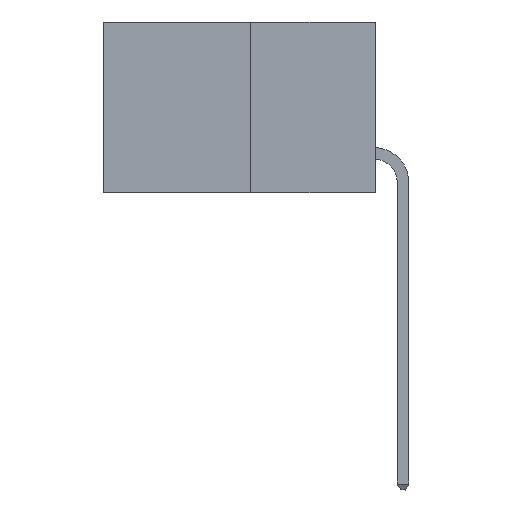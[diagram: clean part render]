
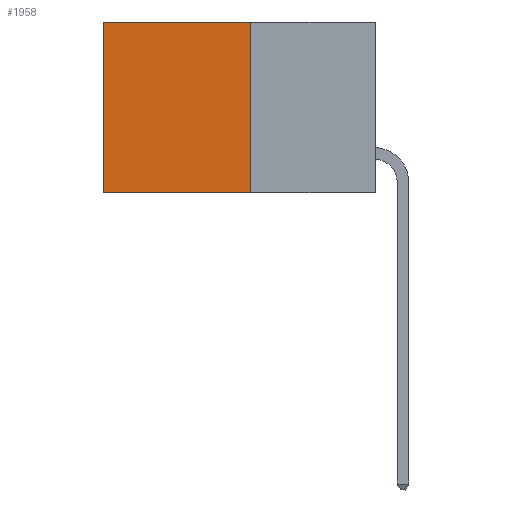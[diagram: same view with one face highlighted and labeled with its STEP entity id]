
A CAD part, left-side view. The second image highlights one B-rep face of the part: STEP entity #1958.
In plain terms, the highlighted planar face has unit normal (-1, 0, 0).
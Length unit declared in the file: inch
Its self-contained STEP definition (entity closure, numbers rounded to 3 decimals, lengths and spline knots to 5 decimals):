
#136 = EDGE_CURVE ( 'NONE', #5969, #7157, #6439, .T. ) ;
#255 = DIRECTION ( 'NONE',  ( 0., 0., -1. ) ) ;
#312 = VECTOR ( 'NONE', #472, 39.37008 ) ;
#472 = DIRECTION ( 'NONE',  ( 0., 0., -1. ) ) ;
#627 = VECTOR ( 'NONE', #8497, 39.37008 ) ;
#854 = VECTOR ( 'NONE', #8159, 39.37008 ) ;
#1305 = LINE ( 'NONE', #4364, #5028 ) ;
#1494 = EDGE_LOOP ( 'NONE', ( #1782, #3955, #5786, #7484 ) ) ;
#1782 = ORIENTED_EDGE ( 'NONE', *, *, #136, .T. ) ;
#1958 = ADVANCED_FACE ( 'NONE', ( #2363 ), #8279, .F. ) ;
#2363 = FACE_OUTER_BOUND ( 'NONE', #1494, .T. ) ;
#2407 = EDGE_CURVE ( 'NONE', #3806, #5969, #3234, .T. ) ;
#2580 = AXIS2_PLACEMENT_3D ( 'NONE', #7180, #4180, #8259 ) ;
#3234 = LINE ( 'NONE', #8153, #854 ) ;
#3716 = CARTESIAN_POINT ( 'NONE',  ( 0.277, 0.27, 0. ) ) ;
#3806 = VERTEX_POINT ( 'NONE', #3716 ) ;
#3955 = ORIENTED_EDGE ( 'NONE', *, *, #9088, .F. ) ;
#4180 = DIRECTION ( 'NONE',  ( 1., 0., 0. ) ) ;
#4364 = CARTESIAN_POINT ( 'NONE',  ( 0.277, 0.27, -0.37 ) ) ;
#4405 = CARTESIAN_POINT ( 'NONE',  ( 0.277, 0.59, -0.37 ) ) ;
#5028 = VECTOR ( 'NONE', #255, 39.37008 ) ;
#5786 = ORIENTED_EDGE ( 'NONE', *, *, #8531, .F. ) ;
#5969 = VERTEX_POINT ( 'NONE', #7809 ) ;
#6439 = LINE ( 'NONE', #4405, #312 ) ;
#7157 = VERTEX_POINT ( 'NONE', #7609 ) ;
#7180 = CARTESIAN_POINT ( 'NONE',  ( 0.277, 0.27, -0.37 ) ) ;
#7231 = VERTEX_POINT ( 'NONE', #8245 ) ;
#7484 = ORIENTED_EDGE ( 'NONE', *, *, #2407, .T. ) ;
#7609 = CARTESIAN_POINT ( 'NONE',  ( 0.277, 0.59, -0.37 ) ) ;
#7809 = CARTESIAN_POINT ( 'NONE',  ( 0.277, 0.59, 0. ) ) ;
#7872 = CARTESIAN_POINT ( 'NONE',  ( 0.277, 0.27, -0.37 ) ) ;
#8153 = CARTESIAN_POINT ( 'NONE',  ( 0.277, 0.27, 0. ) ) ;
#8159 = DIRECTION ( 'NONE',  ( 0., 1., 0. ) ) ;
#8245 = CARTESIAN_POINT ( 'NONE',  ( 0.277, 0.27, -0.37 ) ) ;
#8259 = DIRECTION ( 'NONE',  ( 0., 0., -1. ) ) ;
#8279 = PLANE ( 'NONE',  #2580 ) ;
#8329 = LINE ( 'NONE', #7872, #627 ) ;
#8497 = DIRECTION ( 'NONE',  ( 0., 1., 0. ) ) ;
#8531 = EDGE_CURVE ( 'NONE', #3806, #7231, #1305, .T. ) ;
#9088 = EDGE_CURVE ( 'NONE', #7231, #7157, #8329, .T. ) ;
